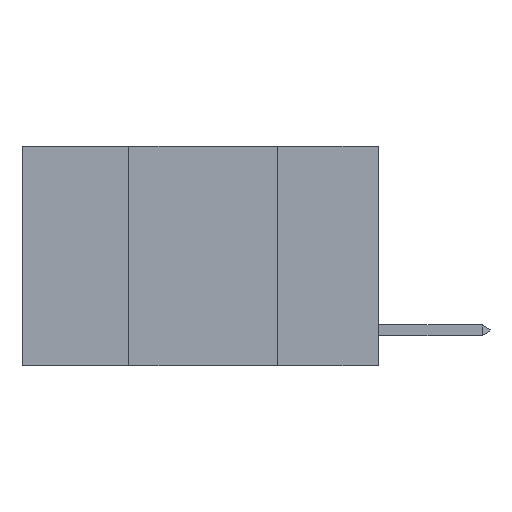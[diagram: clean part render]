
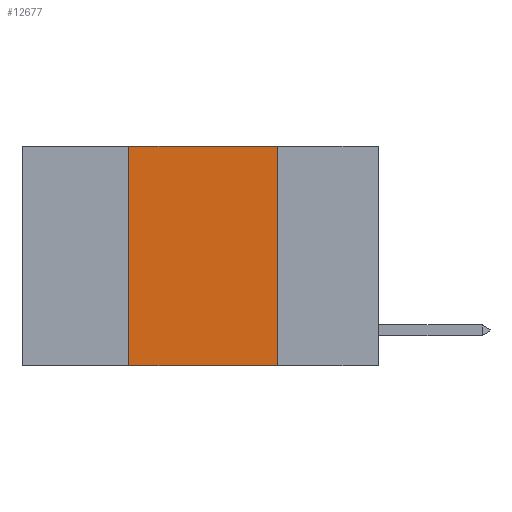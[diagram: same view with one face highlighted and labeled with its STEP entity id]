
A CAD part, left-side view. The second image highlights one B-rep face of the part: STEP entity #12677.
In plain terms, the highlighted planar face has unit normal (-1, 0, 0).
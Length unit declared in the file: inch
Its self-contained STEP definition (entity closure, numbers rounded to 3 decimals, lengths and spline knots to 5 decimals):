
#158 = VERTEX_POINT ( 'NONE', #12169 ) ;
#332 = EDGE_LOOP ( 'NONE', ( #402, #1115, #13536, #9365 ) ) ;
#402 = ORIENTED_EDGE ( 'NONE', *, *, #9667, .F. ) ;
#556 = EDGE_CURVE ( 'NONE', #1165, #11972, #10522, .T. ) ;
#1095 = PLANE ( 'NONE',  #1927 ) ;
#1115 = ORIENTED_EDGE ( 'NONE', *, *, #6441, .F. ) ;
#1165 = VERTEX_POINT ( 'NONE', #8639 ) ;
#1187 = VECTOR ( 'NONE', #2290, 39.37008 ) ;
#1671 = CARTESIAN_POINT ( 'NONE',  ( 0., 0.42, 0. ) ) ;
#1927 = AXIS2_PLACEMENT_3D ( 'NONE', #13878, #11567, #4549 ) ;
#2290 = DIRECTION ( 'NONE',  ( 0., -1., 0. ) ) ;
#3730 = DIRECTION ( 'NONE',  ( 0., -1., 0. ) ) ;
#4549 = DIRECTION ( 'NONE',  ( 0., 0., -1. ) ) ;
#4854 = VERTEX_POINT ( 'NONE', #7705 ) ;
#5145 = FACE_OUTER_BOUND ( 'NONE', #332, .T. ) ;
#5545 = VECTOR ( 'NONE', #3730, 39.37008 ) ;
#6441 = EDGE_CURVE ( 'NONE', #11972, #4854, #13543, .T. ) ;
#6492 = CARTESIAN_POINT ( 'NONE',  ( 0., 0.42, 0. ) ) ;
#7392 = VECTOR ( 'NONE', #13697, 39.37008 ) ;
#7705 = CARTESIAN_POINT ( 'NONE',  ( 0., 0.17, 0. ) ) ;
#8639 = CARTESIAN_POINT ( 'NONE',  ( 0., 0.42, -0.37 ) ) ;
#9365 = ORIENTED_EDGE ( 'NONE', *, *, #10523, .T. ) ;
#9667 = EDGE_CURVE ( 'NONE', #4854, #158, #13868, .T. ) ;
#10522 = LINE ( 'NONE', #1671, #7392 ) ;
#10523 = EDGE_CURVE ( 'NONE', #1165, #158, #14598, .T. ) ;
#10733 = VECTOR ( 'NONE', #10945, 39.37008 ) ;
#10945 = DIRECTION ( 'NONE',  ( 0., 0., -1. ) ) ;
#11567 = DIRECTION ( 'NONE',  ( 1., 0., 0. ) ) ;
#11637 = CARTESIAN_POINT ( 'NONE',  ( 0., 0.6, 0. ) ) ;
#11945 = CARTESIAN_POINT ( 'NONE',  ( 0., 0.6, -0.37 ) ) ;
#11972 = VERTEX_POINT ( 'NONE', #6492 ) ;
#12169 = CARTESIAN_POINT ( 'NONE',  ( 0., 0.17, -0.37 ) ) ;
#12677 = ADVANCED_FACE ( 'NONE', ( #5145 ), #1095, .F. ) ;
#13536 = ORIENTED_EDGE ( 'NONE', *, *, #556, .F. ) ;
#13543 = LINE ( 'NONE', #11637, #1187 ) ;
#13697 = DIRECTION ( 'NONE',  ( 0., 0., 1. ) ) ;
#13868 = LINE ( 'NONE', #14478, #10733 ) ;
#13878 = CARTESIAN_POINT ( 'NONE',  ( 0., 0.6, 0. ) ) ;
#14478 = CARTESIAN_POINT ( 'NONE',  ( 0., 0.17, 0. ) ) ;
#14598 = LINE ( 'NONE', #11945, #5545 ) ;
